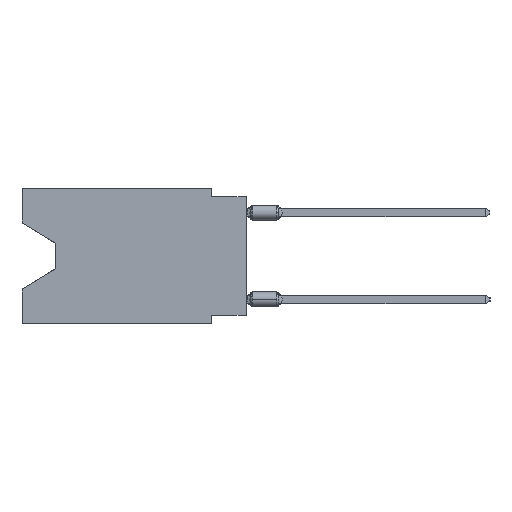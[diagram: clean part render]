
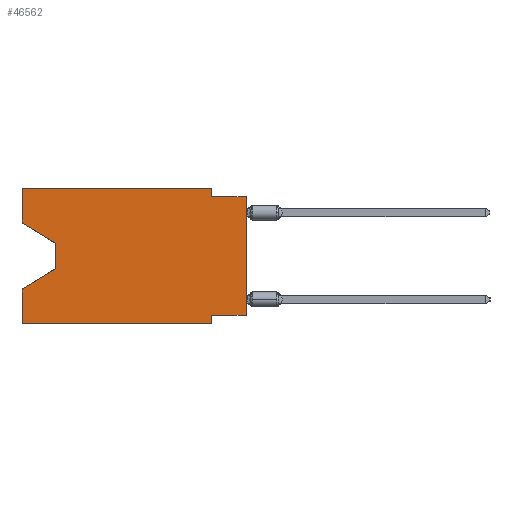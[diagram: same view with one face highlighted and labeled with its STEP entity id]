
A CAD part, left-side view. The second image highlights one B-rep face of the part: STEP entity #46562.
In plain terms, the highlighted planar face has unit normal (-1, 0, 0).
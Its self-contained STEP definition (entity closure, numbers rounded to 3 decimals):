
#97 = DIRECTION ( 'NONE',  ( 0., 0.855, -0.519 ) ) ;
#609 = CARTESIAN_POINT ( 'NONE',  ( 0., 13.97, -4.013 ) ) ;
#795 = EDGE_CURVE ( 'NONE', #14944, #16977, #43972, .T. ) ;
#1404 = LINE ( 'NONE', #49236, #26076 ) ;
#2045 = VERTEX_POINT ( 'NONE', #32964 ) ;
#2289 = ORIENTED_EDGE ( 'NONE', *, *, #39073, .T. ) ;
#2324 = VERTEX_POINT ( 'NONE', #28021 ) ;
#3876 = VERTEX_POINT ( 'NONE', #14152 ) ;
#4388 = DIRECTION ( 'NONE',  ( 0., 0., 1. ) ) ;
#4549 = ORIENTED_EDGE ( 'NONE', *, *, #24330, .F. ) ;
#4717 = DIRECTION ( 'NONE',  ( 0., 0., -1. ) ) ;
#4973 = PLANE ( 'NONE',  #6768 ) ;
#5140 = EDGE_LOOP ( 'NONE', ( #31661, #2289, #38738, #4549, #14453, #34520, #10520, #46434, #18846, #50828, #19248, #15778 ) ) ;
#6531 = VERTEX_POINT ( 'NONE', #13730 ) ;
#6768 = AXIS2_PLACEMENT_3D ( 'NONE', #16313, #31999, #4717 ) ;
#7232 = CARTESIAN_POINT ( 'NONE',  ( 0., 0., 0. ) ) ;
#7400 = VECTOR ( 'NONE', #4388, 1000. ) ;
#7864 = VERTEX_POINT ( 'NONE', #26333 ) ;
#8132 = DIRECTION ( 'NONE',  ( 0., -1., 0. ) ) ;
#8556 = DIRECTION ( 'NONE',  ( 0., 0., -1. ) ) ;
#9935 = EDGE_CURVE ( 'NONE', #6531, #3876, #31497, .T. ) ;
#10133 = VECTOR ( 'NONE', #17947, 1000. ) ;
#10317 = VERTEX_POINT ( 'NONE', #16972 ) ;
#10520 = ORIENTED_EDGE ( 'NONE', *, *, #15472, .F. ) ;
#12387 = VECTOR ( 'NONE', #30406, 1000. ) ;
#12461 = VERTEX_POINT ( 'NONE', #21198 ) ;
#12902 = DIRECTION ( 'NONE',  ( 0., -1., 0. ) ) ;
#13052 = EDGE_CURVE ( 'NONE', #22353, #12461, #43300, .T. ) ;
#13563 = CARTESIAN_POINT ( 'NONE',  ( 0., 0., -0.635 ) ) ;
#13730 = CARTESIAN_POINT ( 'NONE',  ( 0., 16.383, -9.906 ) ) ;
#14024 = DIRECTION ( 'NONE',  ( 0., 0., -1. ) ) ;
#14152 = CARTESIAN_POINT ( 'NONE',  ( 0., 2.54, -9.906 ) ) ;
#14453 = ORIENTED_EDGE ( 'NONE', *, *, #9935, .T. ) ;
#14667 = CARTESIAN_POINT ( 'NONE',  ( 0., 16.383, -2.546 ) ) ;
#14887 = LINE ( 'NONE', #22833, #43054 ) ;
#14944 = VERTEX_POINT ( 'NONE', #37572 ) ;
#15472 = EDGE_CURVE ( 'NONE', #7864, #2324, #14887, .T. ) ;
#15778 = ORIENTED_EDGE ( 'NONE', *, *, #795, .F. ) ;
#16313 = CARTESIAN_POINT ( 'NONE',  ( 0., 16.383, 0. ) ) ;
#16972 = CARTESIAN_POINT ( 'NONE',  ( 0., 2.54, -0.635 ) ) ;
#16977 = VERTEX_POINT ( 'NONE', #24140 ) ;
#17827 = VERTEX_POINT ( 'NONE', #34224 ) ;
#17947 = DIRECTION ( 'NONE',  ( 0., -1., 0. ) ) ;
#18176 = CARTESIAN_POINT ( 'NONE',  ( 0., 13.97, -5.893 ) ) ;
#18846 = ORIENTED_EDGE ( 'NONE', *, *, #24898, .F. ) ;
#19248 = ORIENTED_EDGE ( 'NONE', *, *, #46039, .F. ) ;
#20685 = VECTOR ( 'NONE', #50365, 1000. ) ;
#21198 = CARTESIAN_POINT ( 'NONE',  ( 0., 16.383, -7.36 ) ) ;
#22353 = VERTEX_POINT ( 'NONE', #18176 ) ;
#22833 = CARTESIAN_POINT ( 'NONE',  ( 0., 0., -9.271 ) ) ;
#24140 = CARTESIAN_POINT ( 'NONE',  ( 0., 16.383, 0. ) ) ;
#24265 = EDGE_CURVE ( 'NONE', #7864, #2045, #41968, .T. ) ;
#24330 = EDGE_CURVE ( 'NONE', #6531, #12461, #26287, .T. ) ;
#24898 = EDGE_CURVE ( 'NONE', #10317, #2045, #48278, .T. ) ;
#25000 = VECTOR ( 'NONE', #8556, 1000. ) ;
#26076 = VECTOR ( 'NONE', #14024, 1000. ) ;
#26287 = LINE ( 'NONE', #46569, #41304 ) ;
#26333 = CARTESIAN_POINT ( 'NONE',  ( 0., 0., -9.271 ) ) ;
#26455 = VECTOR ( 'NONE', #8132, 1000. ) ;
#26688 = DIRECTION ( 'NONE',  ( 0., 1., 0. ) ) ;
#26963 = EDGE_CURVE ( 'NONE', #17827, #10317, #28124, .T. ) ;
#27152 = VECTOR ( 'NONE', #97, 1000. ) ;
#27514 = DIRECTION ( 'NONE',  ( 0., 0., -1. ) ) ;
#28021 = CARTESIAN_POINT ( 'NONE',  ( 0., 2.54, -9.271 ) ) ;
#28124 = LINE ( 'NONE', #43796, #25000 ) ;
#30405 = VECTOR ( 'NONE', #27514, 1000. ) ;
#30406 = DIRECTION ( 'NONE',  ( 0., 0., 1. ) ) ;
#31497 = LINE ( 'NONE', #47164, #41703 ) ;
#31661 = ORIENTED_EDGE ( 'NONE', *, *, #44226, .T. ) ;
#31999 = DIRECTION ( 'NONE',  ( 1., 0., 0. ) ) ;
#32530 = EDGE_CURVE ( 'NONE', #2324, #3876, #1404, .T. ) ;
#32964 = CARTESIAN_POINT ( 'NONE',  ( 0., 0., -0.635 ) ) ;
#34224 = CARTESIAN_POINT ( 'NONE',  ( 0., 2.54, 0. ) ) ;
#34520 = ORIENTED_EDGE ( 'NONE', *, *, #32530, .F. ) ;
#35341 = CARTESIAN_POINT ( 'NONE',  ( 0., 13.97, -5.893 ) ) ;
#37092 = VERTEX_POINT ( 'NONE', #609 ) ;
#37572 = CARTESIAN_POINT ( 'NONE',  ( 0., 16.383, -2.546 ) ) ;
#38738 = ORIENTED_EDGE ( 'NONE', *, *, #13052, .T. ) ;
#39073 = EDGE_CURVE ( 'NONE', #37092, #22353, #50168, .T. ) ;
#39630 = CARTESIAN_POINT ( 'NONE',  ( 0., 16.383, 0. ) ) ;
#39759 = LINE ( 'NONE', #47210, #26455 ) ;
#41304 = VECTOR ( 'NONE', #46315, 1000. ) ;
#41703 = VECTOR ( 'NONE', #12902, 1000. ) ;
#41968 = LINE ( 'NONE', #7232, #12387 ) ;
#43054 = VECTOR ( 'NONE', #26688, 1000. ) ;
#43300 = LINE ( 'NONE', #35341, #27152 ) ;
#43457 = CARTESIAN_POINT ( 'NONE',  ( 0., 13.97, -4.013 ) ) ;
#43796 = CARTESIAN_POINT ( 'NONE',  ( 0., 2.54, 0. ) ) ;
#43972 = LINE ( 'NONE', #39630, #7400 ) ;
#44226 = EDGE_CURVE ( 'NONE', #14944, #37092, #49618, .T. ) ;
#44564 = FACE_OUTER_BOUND ( 'NONE', #5140, .T. ) ;
#46039 = EDGE_CURVE ( 'NONE', #16977, #17827, #39759, .T. ) ;
#46315 = DIRECTION ( 'NONE',  ( 0., 0., 1. ) ) ;
#46434 = ORIENTED_EDGE ( 'NONE', *, *, #24265, .T. ) ;
#46562 = ADVANCED_FACE ( 'NONE', ( #44564 ), #4973, .F. ) ;
#46569 = CARTESIAN_POINT ( 'NONE',  ( 0., 16.383, 0. ) ) ;
#47164 = CARTESIAN_POINT ( 'NONE',  ( 0., 16.383, -9.906 ) ) ;
#47210 = CARTESIAN_POINT ( 'NONE',  ( 0., 16.383, 0. ) ) ;
#48278 = LINE ( 'NONE', #13563, #10133 ) ;
#49236 = CARTESIAN_POINT ( 'NONE',  ( 0., 2.54, -9.906 ) ) ;
#49618 = LINE ( 'NONE', #14667, #20685 ) ;
#50168 = LINE ( 'NONE', #43457, #30405 ) ;
#50365 = DIRECTION ( 'NONE',  ( 0., -0.855, -0.519 ) ) ;
#50828 = ORIENTED_EDGE ( 'NONE', *, *, #26963, .F. ) ;
